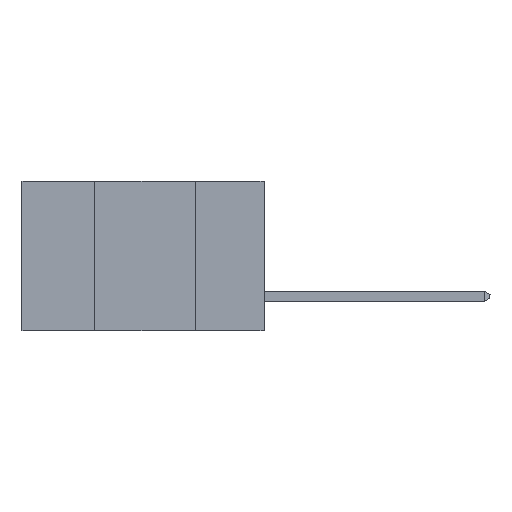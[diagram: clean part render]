
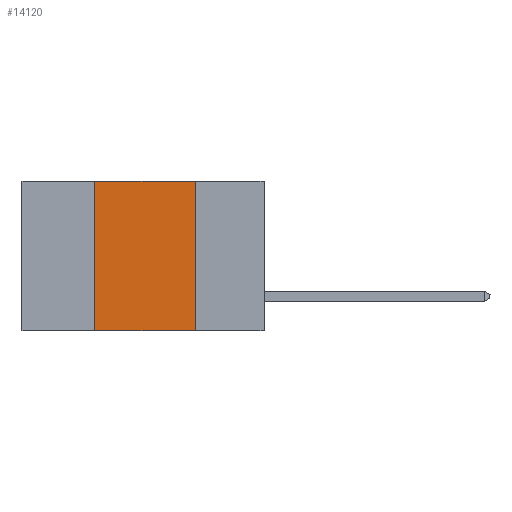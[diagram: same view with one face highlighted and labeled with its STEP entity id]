
A CAD part, left-side view. The second image highlights one B-rep face of the part: STEP entity #14120.
In plain terms, the highlighted planar face has unit normal (-1, 0, 0).
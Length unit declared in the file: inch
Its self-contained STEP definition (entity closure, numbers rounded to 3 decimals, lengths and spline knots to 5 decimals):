
#652 = VECTOR ( 'NONE', #13010, 39.37008 ) ;
#974 = VECTOR ( 'NONE', #12813, 39.37008 ) ;
#1489 = AXIS2_PLACEMENT_3D ( 'NONE', #2569, #13070, #10467 ) ;
#1613 = LINE ( 'NONE', #3909, #652 ) ;
#2145 = CARTESIAN_POINT ( 'NONE',  ( 0., 0.6, 0. ) ) ;
#2170 = CARTESIAN_POINT ( 'NONE',  ( 0., 0.42, -0.37 ) ) ;
#2569 = CARTESIAN_POINT ( 'NONE',  ( 0., 0.6, 0. ) ) ;
#3909 = CARTESIAN_POINT ( 'NONE',  ( 0., 0.6, -0.37 ) ) ;
#4457 = LINE ( 'NONE', #2170, #14343 ) ;
#4561 = ORIENTED_EDGE ( 'NONE', *, *, #10745, .F. ) ;
#4581 = VERTEX_POINT ( 'NONE', #14060 ) ;
#4587 = EDGE_CURVE ( 'NONE', #4581, #12722, #1613, .T. ) ;
#4848 = ORIENTED_EDGE ( 'NONE', *, *, #10545, .F. ) ;
#5648 = LINE ( 'NONE', #2145, #6461 ) ;
#6461 = VECTOR ( 'NONE', #6625, 39.37008 ) ;
#6625 = DIRECTION ( 'NONE',  ( 0., -1., 0. ) ) ;
#6733 = VERTEX_POINT ( 'NONE', #7423 ) ;
#7278 = PLANE ( 'NONE',  #1489 ) ;
#7317 = EDGE_LOOP ( 'NONE', ( #4848, #4561, #8269, #13354 ) ) ;
#7423 = CARTESIAN_POINT ( 'NONE',  ( 0., 0.17, 0. ) ) ;
#7802 = CARTESIAN_POINT ( 'NONE',  ( 0., 0.17, -0.37 ) ) ;
#8269 = ORIENTED_EDGE ( 'NONE', *, *, #14273, .F. ) ;
#9111 = VERTEX_POINT ( 'NONE', #12501 ) ;
#9168 = LINE ( 'NONE', #9455, #974 ) ;
#9455 = CARTESIAN_POINT ( 'NONE',  ( 0., 0.17, -0.37 ) ) ;
#10132 = DIRECTION ( 'NONE',  ( 0., 0., 1. ) ) ;
#10467 = DIRECTION ( 'NONE',  ( 0., 0., -1. ) ) ;
#10545 = EDGE_CURVE ( 'NONE', #6733, #12722, #9168, .T. ) ;
#10745 = EDGE_CURVE ( 'NONE', #9111, #6733, #5648, .T. ) ;
#11893 = FACE_OUTER_BOUND ( 'NONE', #7317, .T. ) ;
#12501 = CARTESIAN_POINT ( 'NONE',  ( 0., 0.42, 0. ) ) ;
#12722 = VERTEX_POINT ( 'NONE', #7802 ) ;
#12813 = DIRECTION ( 'NONE',  ( 0., 0., -1. ) ) ;
#13010 = DIRECTION ( 'NONE',  ( 0., -1., 0. ) ) ;
#13070 = DIRECTION ( 'NONE',  ( 1., 0., 0. ) ) ;
#13354 = ORIENTED_EDGE ( 'NONE', *, *, #4587, .T. ) ;
#14060 = CARTESIAN_POINT ( 'NONE',  ( 0., 0.42, -0.37 ) ) ;
#14120 = ADVANCED_FACE ( 'NONE', ( #11893 ), #7278, .F. ) ;
#14273 = EDGE_CURVE ( 'NONE', #4581, #9111, #4457, .T. ) ;
#14343 = VECTOR ( 'NONE', #10132, 39.37008 ) ;
